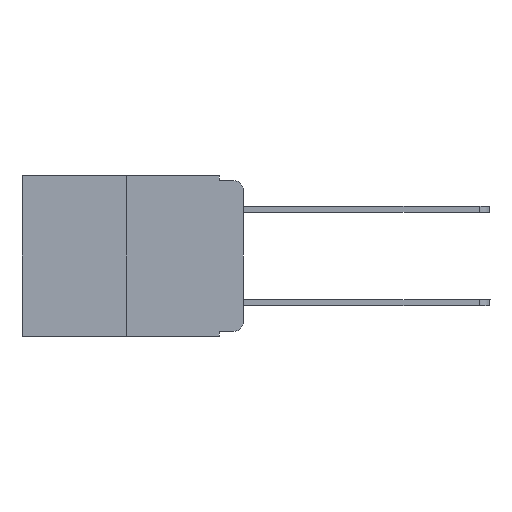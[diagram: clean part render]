
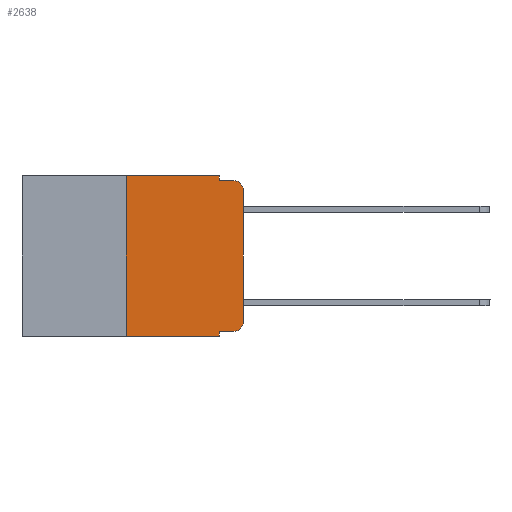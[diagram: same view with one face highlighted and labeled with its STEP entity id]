
A CAD part, left-side view. The second image highlights one B-rep face of the part: STEP entity #2638.
In plain terms, the highlighted planar face has unit normal (-1, 0, 0).
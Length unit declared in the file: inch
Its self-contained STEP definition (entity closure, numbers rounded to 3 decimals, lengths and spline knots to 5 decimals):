
#375 = DIRECTION ( 'NONE',  ( 0., 0., -1. ) ) ;
#485 = CARTESIAN_POINT ( 'NONE',  ( 0., 0.02, -0.03 ) ) ;
#671 = EDGE_CURVE ( 'NONE', #12849, #9357, #11233, .T. ) ;
#701 = DIRECTION ( 'NONE',  ( 0., -1., 0. ) ) ;
#725 = ORIENTED_EDGE ( 'NONE', *, *, #3299, .F. ) ;
#1090 = CARTESIAN_POINT ( 'NONE',  ( 0., 0.02, -0.313 ) ) ;
#1141 = VECTOR ( 'NONE', #6664, 39.37008 ) ;
#1143 = EDGE_CURVE ( 'NONE', #9357, #10187, #1408, .T. ) ;
#1146 = CARTESIAN_POINT ( 'NONE',  ( 0., 0.02, -0.333 ) ) ;
#1408 = LINE ( 'NONE', #12679, #4960 ) ;
#1470 = EDGE_CURVE ( 'NONE', #11073, #10187, #5430, .T. ) ;
#2277 = DIRECTION ( 'NONE',  ( 0., 0., -1. ) ) ;
#2501 = LINE ( 'NONE', #8670, #12551 ) ;
#2554 = ORIENTED_EDGE ( 'NONE', *, *, #5203, .T. ) ;
#2638 = ADVANCED_FACE ( 'NONE', ( #10656 ), #10987, .F. ) ;
#2769 = DIRECTION ( 'NONE',  ( 0., -1., 0. ) ) ;
#2961 = ORIENTED_EDGE ( 'NONE', *, *, #12672, .T. ) ;
#2976 = LINE ( 'NONE', #8653, #11781 ) ;
#3082 = ORIENTED_EDGE ( 'NONE', *, *, #13180, .T. ) ;
#3273 = VECTOR ( 'NONE', #375, 39.37008 ) ;
#3299 = EDGE_CURVE ( 'NONE', #7999, #12849, #13135, .T. ) ;
#3356 = AXIS2_PLACEMENT_3D ( 'NONE', #1090, #12833, #6357 ) ;
#3734 = CARTESIAN_POINT ( 'NONE',  ( 0., 0.051, -0.01 ) ) ;
#3767 = EDGE_LOOP ( 'NONE', ( #2961, #11422, #8304, #11286, #725, #13565, #3082, #5467, #12351, #2554 ) ) ;
#3911 = CARTESIAN_POINT ( 'NONE',  ( 0., 0., 0. ) ) ;
#3971 = AXIS2_PLACEMENT_3D ( 'NONE', #485, #5785, #11307 ) ;
#4647 = CARTESIAN_POINT ( 'NONE',  ( 0., 0.473, -0.343 ) ) ;
#4926 = VERTEX_POINT ( 'NONE', #6969 ) ;
#4960 = VECTOR ( 'NONE', #701, 39.37008 ) ;
#4996 = CARTESIAN_POINT ( 'NONE',  ( 0., 0., -0.03 ) ) ;
#5145 = VECTOR ( 'NONE', #2769, 39.37008 ) ;
#5203 = EDGE_CURVE ( 'NONE', #9809, #12423, #13632, .T. ) ;
#5350 = EDGE_CURVE ( 'NONE', #4926, #9809, #2976, .T. ) ;
#5430 = CIRCLE ( 'NONE', #3971, 0.02 ) ;
#5467 = ORIENTED_EDGE ( 'NONE', *, *, #6939, .F. ) ;
#5785 = DIRECTION ( 'NONE',  ( -1., 0., 0. ) ) ;
#6182 = LINE ( 'NONE', #4647, #1141 ) ;
#6357 = DIRECTION ( 'NONE',  ( 0., 0., -1. ) ) ;
#6664 = DIRECTION ( 'NONE',  ( 0., -1., 0. ) ) ;
#6728 = LINE ( 'NONE', #7131, #13536 ) ;
#6939 = EDGE_CURVE ( 'NONE', #4926, #10157, #2501, .T. ) ;
#6969 = CARTESIAN_POINT ( 'NONE',  ( 0., 0.051, -0.333 ) ) ;
#7060 = CARTESIAN_POINT ( 'NONE',  ( 0., 0.473, 0. ) ) ;
#7104 = DIRECTION ( 'NONE',  ( 0., 0., 1. ) ) ;
#7131 = CARTESIAN_POINT ( 'NONE',  ( 0., 0.25, 0. ) ) ;
#7133 = VERTEX_POINT ( 'NONE', #13768 ) ;
#7551 = LINE ( 'NONE', #3911, #9401 ) ;
#7613 = CARTESIAN_POINT ( 'NONE',  ( 0., 0.473, 0. ) ) ;
#7661 = DIRECTION ( 'NONE',  ( 1., 0., 0. ) ) ;
#7999 = VERTEX_POINT ( 'NONE', #10070 ) ;
#8304 = ORIENTED_EDGE ( 'NONE', *, *, #1143, .F. ) ;
#8653 = CARTESIAN_POINT ( 'NONE',  ( 0., 0.051, -0.333 ) ) ;
#8670 = CARTESIAN_POINT ( 'NONE',  ( 0., 0.051, 0. ) ) ;
#9199 = AXIS2_PLACEMENT_3D ( 'NONE', #7613, #7661, #2277 ) ;
#9225 = CARTESIAN_POINT ( 'NONE',  ( 0., 0.02, -0.01 ) ) ;
#9357 = VERTEX_POINT ( 'NONE', #3734 ) ;
#9401 = VECTOR ( 'NONE', #7104, 39.37008 ) ;
#9809 = VERTEX_POINT ( 'NONE', #1146 ) ;
#10070 = CARTESIAN_POINT ( 'NONE',  ( 0., 0.25, 0. ) ) ;
#10157 = VERTEX_POINT ( 'NONE', #10273 ) ;
#10187 = VERTEX_POINT ( 'NONE', #9225 ) ;
#10273 = CARTESIAN_POINT ( 'NONE',  ( 0., 0.051, -0.343 ) ) ;
#10656 = FACE_OUTER_BOUND ( 'NONE', #3767, .T. ) ;
#10871 = DIRECTION ( 'NONE',  ( 0., 0., -1. ) ) ;
#10987 = PLANE ( 'NONE',  #9199 ) ;
#11073 = VERTEX_POINT ( 'NONE', #4996 ) ;
#11233 = LINE ( 'NONE', #11262, #3273 ) ;
#11262 = CARTESIAN_POINT ( 'NONE',  ( 0., 0.051, 0. ) ) ;
#11286 = ORIENTED_EDGE ( 'NONE', *, *, #671, .F. ) ;
#11307 = DIRECTION ( 'NONE',  ( 0., 0., -1. ) ) ;
#11422 = ORIENTED_EDGE ( 'NONE', *, *, #1470, .T. ) ;
#11601 = CARTESIAN_POINT ( 'NONE',  ( 0., 0., -0.313 ) ) ;
#11650 = EDGE_CURVE ( 'NONE', #7133, #7999, #6728, .T. ) ;
#11781 = VECTOR ( 'NONE', #12003, 39.37008 ) ;
#12003 = DIRECTION ( 'NONE',  ( 0., -1., 0. ) ) ;
#12351 = ORIENTED_EDGE ( 'NONE', *, *, #5350, .T. ) ;
#12423 = VERTEX_POINT ( 'NONE', #11601 ) ;
#12551 = VECTOR ( 'NONE', #10871, 39.37008 ) ;
#12621 = DIRECTION ( 'NONE',  ( 0., 0., 1. ) ) ;
#12672 = EDGE_CURVE ( 'NONE', #12423, #11073, #7551, .T. ) ;
#12679 = CARTESIAN_POINT ( 'NONE',  ( 0., 0.051, -0.01 ) ) ;
#12784 = CARTESIAN_POINT ( 'NONE',  ( 0., 0.051, 0. ) ) ;
#12833 = DIRECTION ( 'NONE',  ( -1., 0., 0. ) ) ;
#12849 = VERTEX_POINT ( 'NONE', #12784 ) ;
#13135 = LINE ( 'NONE', #7060, #5145 ) ;
#13180 = EDGE_CURVE ( 'NONE', #7133, #10157, #6182, .T. ) ;
#13536 = VECTOR ( 'NONE', #12621, 39.37008 ) ;
#13565 = ORIENTED_EDGE ( 'NONE', *, *, #11650, .F. ) ;
#13632 = CIRCLE ( 'NONE', #3356, 0.02 ) ;
#13768 = CARTESIAN_POINT ( 'NONE',  ( 0., 0.25, -0.343 ) ) ;
